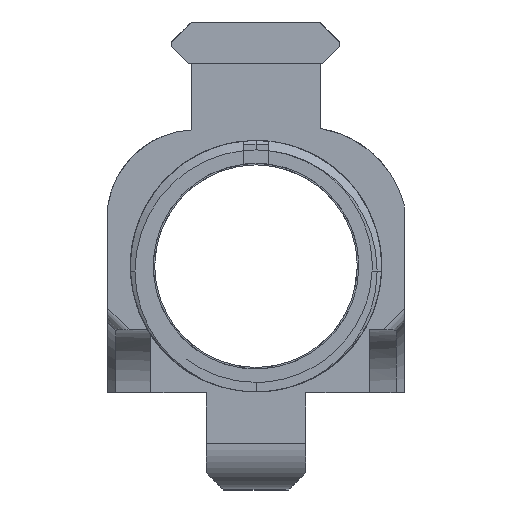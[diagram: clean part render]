
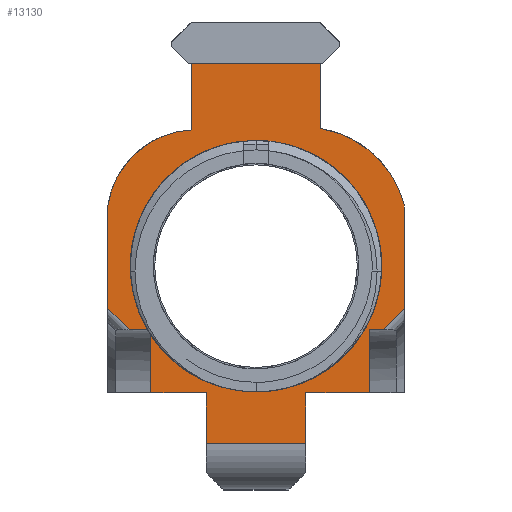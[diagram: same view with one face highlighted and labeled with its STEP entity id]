
A CAD part, front view. The second image highlights one B-rep face of the part: STEP entity #13130.
In plain terms, the highlighted planar face has unit normal (0, -1, 0).
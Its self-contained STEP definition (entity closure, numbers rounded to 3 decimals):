
#96=FACE_BOUND('',#2438,.T.);
#512=CIRCLE('',#13183,13.139);
#664=CIRCLE('',#13837,11.274);
#674=CIRCLE('',#13882,14.891);
#1060=PLANE('',#13883);
#1730=FACE_OUTER_BOUND('',#2437,.T.);
#2437=EDGE_LOOP('',(#12226,#12227,#12228,#12229,#12230,#12231,#12232,#12233,
#12234,#12235,#12236,#12237,#12238,#12239,#12240,#12241,#12242,#12243,#12244,
#12245));
#2438=EDGE_LOOP('',(#12246));
#2543=B_SPLINE_CURVE_WITH_KNOTS('',3,(#19589,#19590,#19591,#19592),
 .UNSPECIFIED.,.F.,.F.,(4,4),(0.181,0.554),
 .UNSPECIFIED.);
#2624=B_SPLINE_CURVE_WITH_KNOTS('',3,(#22441,#22442,#22443,#22444),
 .UNSPECIFIED.,.F.,.F.,(4,4),(2.069,2.456),
 .UNSPECIFIED.);
#2695=LINE('',#17619,#3991);
#2712=LINE('',#17660,#4008);
#3067=LINE('',#20091,#4363);
#3094=LINE('',#20266,#4390);
#3176=LINE('',#20441,#4472);
#3386=LINE('',#21311,#4682);
#3559=LINE('',#22309,#4855);
#3561=LINE('',#22314,#4857);
#3563=LINE('',#22320,#4859);
#3565=LINE('',#22324,#4861);
#3571=LINE('',#22347,#4867);
#3572=LINE('',#22349,#4868);
#3578=LINE('',#22386,#4874);
#3923=LINE('',#24585,#5219);
#3961=LINE('',#25352,#5257);
#3962=LINE('',#25353,#5258);
#3991=VECTOR('',#13972,10.);
#4008=VECTOR('',#13999,10.);
#4363=VECTOR('',#14652,10.);
#4390=VECTOR('',#14751,10.);
#4472=VECTOR('',#14859,10.);
#4682=VECTOR('',#15337,12.548);
#4855=VECTOR('',#15856,10.);
#4857=VECTOR('',#15862,10.);
#4859=VECTOR('',#15868,10.);
#4861=VECTOR('',#15872,10.);
#4867=VECTOR('',#15888,10.);
#4868=VECTOR('',#15889,10.);
#4874=VECTOR('',#15897,10.);
#5219=VECTOR('',#16492,10.);
#5257=VECTOR('',#16626,10.);
#5258=VECTOR('',#16627,10.);
#5324=VERTEX_POINT('',#17496);
#5325=VERTEX_POINT('',#17498);
#5332=VERTEX_POINT('',#17618);
#5351=VERTEX_POINT('',#17658);
#5709=VERTEX_POINT('',#19577);
#5710=VERTEX_POINT('',#19588);
#5737=VERTEX_POINT('',#20089);
#5738=VERTEX_POINT('',#20090);
#5787=VERTEX_POINT('',#20264);
#5788=VERTEX_POINT('',#20265);
#5867=VERTEX_POINT('',#20439);
#5868=VERTEX_POINT('',#20440);
#6145=VERTEX_POINT('',#22313);
#6147=VERTEX_POINT('',#22319);
#6148=VERTEX_POINT('',#22323);
#6157=VERTEX_POINT('',#22348);
#6164=VERTEX_POINT('',#22385);
#6167=VERTEX_POINT('',#22417);
#6168=VERTEX_POINT('',#22428);
#6512=VERTEX_POINT('',#24584);
#6549=VERTEX_POINT('',#25348);
#6613=EDGE_CURVE('',#5325,#5324,#512,.T.);
#6625=EDGE_CURVE('',#5332,#5325,#2695,.T.);
#6646=EDGE_CURVE('',#5324,#5351,#2712,.F.);
#7137=EDGE_CURVE('',#5709,#5710,#2543,.T.);
#7174=EDGE_CURVE('',#5737,#5738,#3067,.F.);
#7234=EDGE_CURVE('',#5787,#5788,#3094,.T.);
#7322=EDGE_CURVE('',#5867,#5868,#3176,.F.);
#7580=EDGE_CURVE('',#5738,#5867,#3386,.T.);
#7839=EDGE_CURVE('',#5709,#5332,#3559,.T.);
#7842=EDGE_CURVE('',#6145,#5710,#3561,.T.);
#7845=EDGE_CURVE('',#6147,#6145,#3563,.T.);
#7847=EDGE_CURVE('',#6148,#6147,#3565,.T.);
#7858=EDGE_CURVE('',#6148,#5868,#3571,.T.);
#7859=EDGE_CURVE('',#5737,#6157,#3572,.T.);
#7868=EDGE_CURVE('',#6164,#6157,#3578,.T.);
#7875=EDGE_CURVE('',#6168,#6167,#2624,.T.);
#8393=EDGE_CURVE('',#6167,#6512,#3923,.T.);
#8398=EDGE_CURVE('',#5787,#6512,#664,.T.);
#8480=EDGE_CURVE('',#6549,#6549,#674,.T.);
#8481=EDGE_CURVE('',#5351,#5788,#3961,.T.);
#8482=EDGE_CURVE('',#6168,#6164,#3962,.T.);
#12226=ORIENTED_EDGE('',*,*,#8481,.T.);
#12227=ORIENTED_EDGE('',*,*,#7234,.F.);
#12228=ORIENTED_EDGE('',*,*,#8398,.T.);
#12229=ORIENTED_EDGE('',*,*,#8393,.F.);
#12230=ORIENTED_EDGE('',*,*,#7875,.F.);
#12231=ORIENTED_EDGE('',*,*,#8482,.T.);
#12232=ORIENTED_EDGE('',*,*,#7868,.T.);
#12233=ORIENTED_EDGE('',*,*,#7859,.F.);
#12234=ORIENTED_EDGE('',*,*,#7174,.T.);
#12235=ORIENTED_EDGE('',*,*,#7580,.T.);
#12236=ORIENTED_EDGE('',*,*,#7322,.T.);
#12237=ORIENTED_EDGE('',*,*,#7858,.F.);
#12238=ORIENTED_EDGE('',*,*,#7847,.T.);
#12239=ORIENTED_EDGE('',*,*,#7845,.T.);
#12240=ORIENTED_EDGE('',*,*,#7842,.T.);
#12241=ORIENTED_EDGE('',*,*,#7137,.F.);
#12242=ORIENTED_EDGE('',*,*,#7839,.T.);
#12243=ORIENTED_EDGE('',*,*,#6625,.T.);
#12244=ORIENTED_EDGE('',*,*,#6613,.T.);
#12245=ORIENTED_EDGE('',*,*,#6646,.T.);
#12246=ORIENTED_EDGE('',*,*,#8480,.T.);
#13130=ADVANCED_FACE('',(#1730,#96),#1060,.F.);
#13183=AXIS2_PLACEMENT_3D('',#17499,#13954,#13955);
#13837=AXIS2_PLACEMENT_3D('',#24600,#16497,#16498);
#13882=AXIS2_PLACEMENT_3D('',#25350,#16622,#16623);
#13883=AXIS2_PLACEMENT_3D('',#25351,#16624,#16625);
#13954=DIRECTION('center_axis',(0.,-1.,0.));
#13955=DIRECTION('ref_axis',(0.967,0.,0.253));
#13972=DIRECTION('',(0.,0.,1.));
#13999=DIRECTION('',(0.,0.,-1.));
#14652=DIRECTION('',(0.,0.,1.));
#14751=DIRECTION('',(0.,0.,1.));
#14859=DIRECTION('',(0.,0.,-1.));
#15337=DIRECTION('',(1.,0.,0.));
#15856=DIRECTION('',(0.,0.,1.));
#15862=DIRECTION('',(1.,0.,0.));
#15868=DIRECTION('',(0.,0.,1.));
#15872=DIRECTION('',(1.,0.,0.));
#15888=DIRECTION('',(-1.,0.,0.));
#15889=DIRECTION('',(-1.,0.,0.));
#15897=DIRECTION('',(0.,0.,-1.));
#16492=DIRECTION('',(0.,0.,1.));
#16497=DIRECTION('center_axis',(0.,-1.,0.));
#16498=DIRECTION('ref_axis',(-0.049,0.,0.999));
#16622=DIRECTION('center_axis',(0.,1.,0.));
#16623=DIRECTION('ref_axis',(1.,0.,0.));
#16624=DIRECTION('center_axis',(0.,1.,0.));
#16625=DIRECTION('ref_axis',(-1.,0.,0.));
#16626=DIRECTION('',(-1.,0.,0.));
#16627=DIRECTION('',(1.,0.,0.));
#17496=CARTESIAN_POINT('',(8.084,-129.325,-13.951));
#17498=CARTESIAN_POINT('',(18.673,-129.325,-23.592));
#17499=CARTESIAN_POINT('Origin',(5.962,-129.325,-26.918));
#17618=CARTESIAN_POINT('',(18.673,-129.325,-25.966));
#17619=CARTESIAN_POINT('',(18.673,-129.325,-25.966));
#17658=CARTESIAN_POINT('',(8.084,-129.325,-5.736));
#17660=CARTESIAN_POINT('',(8.084,-129.325,-32.048));
#19577=CARTESIAN_POINT('',(18.673,-129.325,-36.646));
#19588=CARTESIAN_POINT('',(16.057,-129.325,-39.312));
#19589=CARTESIAN_POINT('Ctrl Pts',(18.673,-129.325,-36.646));
#19590=CARTESIAN_POINT('Ctrl Pts',(17.8,-129.325,-37.533));
#19591=CARTESIAN_POINT('Ctrl Pts',(16.927,-129.325,-38.421));
#19592=CARTESIAN_POINT('Ctrl Pts',(16.057,-129.325,-39.312));
#20089=CARTESIAN_POINT('',(-6.28,-129.325,-47.288));
#20090=CARTESIAN_POINT('',(-6.28,-129.325,-53.638));
#20091=CARTESIAN_POINT('',(-6.28,-129.325,-55.492));
#20264=CARTESIAN_POINT('',(-8.096,-129.325,-14.13));
#20265=CARTESIAN_POINT('',(-8.096,-129.325,-5.736));
#20266=CARTESIAN_POINT('',(-8.096,-129.325,-35.522));
#20439=CARTESIAN_POINT('',(6.267,-129.325,-53.638));
#20440=CARTESIAN_POINT('',(6.267,-129.325,-47.288));
#20441=CARTESIAN_POINT('',(6.267,-129.325,-50.463));
#21311=CARTESIAN_POINT('',(-6.28,-129.325,-53.638));
#22309=CARTESIAN_POINT('',(18.673,-129.325,-47.288));
#22313=CARTESIAN_POINT('',(14.288,-129.325,-39.312));
#22314=CARTESIAN_POINT('',(18.673,-129.325,-39.312));
#22319=CARTESIAN_POINT('',(14.287,-129.325,-47.288));
#22320=CARTESIAN_POINT('',(14.287,-129.325,-45.132));
#22323=CARTESIAN_POINT('',(11.106,-129.325,-47.288));
#22324=CARTESIAN_POINT('',(11.106,-129.325,-47.288));
#22347=CARTESIAN_POINT('',(-14.862,-129.325,-47.288));
#22348=CARTESIAN_POINT('',(-13.259,-129.325,-47.288));
#22349=CARTESIAN_POINT('',(-7.44,-129.325,-47.288));
#22385=CARTESIAN_POINT('',(-13.259,-129.325,-39.331));
#22386=CARTESIAN_POINT('',(-13.259,-129.325,-44.569));
#22417=CARTESIAN_POINT('',(-18.696,-129.325,-36.583));
#22428=CARTESIAN_POINT('',(-15.966,-129.325,-39.331));
#22441=CARTESIAN_POINT('Ctrl Pts',(-15.966,-129.325,
-39.331));
#22442=CARTESIAN_POINT('Ctrl Pts',(-16.875,-129.325,-38.414));
#22443=CARTESIAN_POINT('Ctrl Pts',(-17.785,-129.325,
-37.498));
#22444=CARTESIAN_POINT('Ctrl Pts',(-18.696,-129.325,
-36.583));
#24584=CARTESIAN_POINT('',(-18.696,-129.325,-23.71));
#24585=CARTESIAN_POINT('',(-18.696,-129.325,-47.288));
#24600=CARTESIAN_POINT('Origin',(-7.548,-129.325,-25.39));
#25348=CARTESIAN_POINT('',(-14.897,-129.325,-31.311));
#25350=CARTESIAN_POINT('Origin',(-0.006,-129.325,
-31.311));
#25351=CARTESIAN_POINT('Origin',(-15.43,-129.325,-53.638));
#25352=CARTESIAN_POINT('',(-11.979,-129.325,-5.736));
#25353=CARTESIAN_POINT('',(-18.696,-129.325,-39.331));
